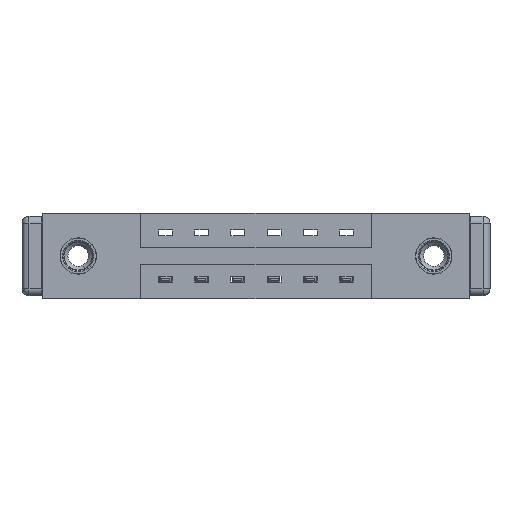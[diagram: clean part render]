
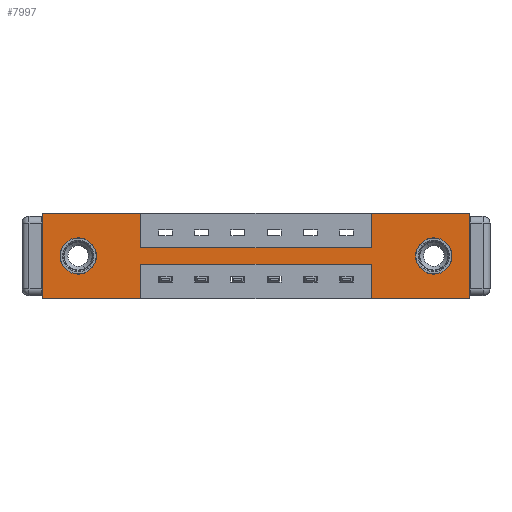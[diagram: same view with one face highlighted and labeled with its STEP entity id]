
A CAD part, front view. The second image highlights one B-rep face of the part: STEP entity #7997.
In plain terms, the highlighted planar face has unit normal (0, -1, 0).
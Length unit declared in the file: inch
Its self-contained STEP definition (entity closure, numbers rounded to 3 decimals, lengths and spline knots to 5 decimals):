
#38 = EDGE_CURVE ( 'NONE', #2394, #8816, #233, .T. ) ;
#136 = DIRECTION ( 'NONE',  ( 1., 0., 0. ) ) ;
#142 = DIRECTION ( 'NONE',  ( 0., 0., -1. ) ) ;
#158 = PLANE ( 'NONE',  #6622 ) ;
#172 = ORIENTED_EDGE ( 'NONE', *, *, #10269, .F. ) ;
#233 = LINE ( 'NONE', #5100, #368 ) ;
#368 = VECTOR ( 'NONE', #636, 39.37008 ) ;
#400 = VECTOR ( 'NONE', #8932, 39.37008 ) ;
#459 = CIRCLE ( 'NONE', #5070, 0.078 ) ;
#519 = ORIENTED_EDGE ( 'NONE', *, *, #772, .T. ) ;
#539 = ORIENTED_EDGE ( 'NONE', *, *, #7201, .F. ) ;
#636 = DIRECTION ( 'NONE',  ( 0., 0., 1. ) ) ;
#690 = VERTEX_POINT ( 'NONE', #1892 ) ;
#763 = DIRECTION ( 'NONE',  ( 0., 1., 0. ) ) ;
#772 = EDGE_CURVE ( 'NONE', #3120, #1529, #9039, .T. ) ;
#1170 = CARTESIAN_POINT ( 'NONE',  ( 0.425, 0., 0. ) ) ;
#1273 = ORIENTED_EDGE ( 'NONE', *, *, #7797, .F. ) ;
#1277 = ORIENTED_EDGE ( 'NONE', *, *, #1771, .F. ) ;
#1303 = ORIENTED_EDGE ( 'NONE', *, *, #38, .F. ) ;
#1448 = ORIENTED_EDGE ( 'NONE', *, *, #5580, .F. ) ;
#1529 = VERTEX_POINT ( 'NONE', #10705 ) ;
#1572 = DIRECTION ( 'NONE',  ( -1., 0., 0. ) ) ;
#1639 = CARTESIAN_POINT ( 'NONE',  ( 1.417, 0., -0.15 ) ) ;
#1703 = VERTEX_POINT ( 'NONE', #2415 ) ;
#1771 = EDGE_CURVE ( 'NONE', #8816, #7297, #5642, .T. ) ;
#1779 = CARTESIAN_POINT ( 'NONE',  ( 0., 0., 0. ) ) ;
#1783 = CARTESIAN_POINT ( 'NONE',  ( 0.425, 0., -0.15 ) ) ;
#1792 = FACE_BOUND ( 'NONE', #9631, .T. ) ;
#1835 = DIRECTION ( 'NONE',  ( 0., 0., -1. ) ) ;
#1892 = CARTESIAN_POINT ( 'NONE',  ( 0.155, 0., -0.107 ) ) ;
#1911 = EDGE_CURVE ( 'NONE', #3802, #2394, #8894, .T. ) ;
#1972 = CARTESIAN_POINT ( 'NONE',  ( 1.687, 0., -0.185 ) ) ;
#2100 = CARTESIAN_POINT ( 'NONE',  ( 0., 0., 0. ) ) ;
#2121 = VERTEX_POINT ( 'NONE', #7579 ) ;
#2150 = DIRECTION ( 'NONE',  ( 0., 0., 1. ) ) ;
#2299 = LINE ( 'NONE', #6321, #2576 ) ;
#2394 = VERTEX_POINT ( 'NONE', #1639 ) ;
#2415 = CARTESIAN_POINT ( 'NONE',  ( 1.417, 0., -0.37 ) ) ;
#2576 = VECTOR ( 'NONE', #3611, 39.37008 ) ;
#2641 = DIRECTION ( 'NONE',  ( 0., 0., -1. ) ) ;
#2748 = DIRECTION ( 'NONE',  ( 0., -1., 0. ) ) ;
#2850 = VERTEX_POINT ( 'NONE', #1170 ) ;
#2863 = DIRECTION ( 'NONE',  ( 0., 0., -1. ) ) ;
#3120 = VERTEX_POINT ( 'NONE', #9596 ) ;
#3240 = LINE ( 'NONE', #4805, #9347 ) ;
#3254 = LINE ( 'NONE', #8223, #7430 ) ;
#3289 = CARTESIAN_POINT ( 'NONE',  ( 0., 0., -0.37 ) ) ;
#3500 = CARTESIAN_POINT ( 'NONE',  ( 1.687, 0., -0.185 ) ) ;
#3555 = DIRECTION ( 'NONE',  ( 0., 0., 1. ) ) ;
#3592 = CARTESIAN_POINT ( 'NONE',  ( 0.425, 0., -0.37 ) ) ;
#3610 = VECTOR ( 'NONE', #8745, 39.37008 ) ;
#3611 = DIRECTION ( 'NONE',  ( -1., 0., 0. ) ) ;
#3703 = ORIENTED_EDGE ( 'NONE', *, *, #1911, .F. ) ;
#3747 = CARTESIAN_POINT ( 'NONE',  ( 0., 0., 0. ) ) ;
#3802 = VERTEX_POINT ( 'NONE', #10780 ) ;
#3962 = LINE ( 'NONE', #3289, #5983 ) ;
#4008 = CARTESIAN_POINT ( 'NONE',  ( 1.417, 0., -0.37 ) ) ;
#4165 = CARTESIAN_POINT ( 'NONE',  ( 1.417, 0., 0. ) ) ;
#4197 = LINE ( 'NONE', #4008, #3610 ) ;
#4304 = EDGE_CURVE ( 'NONE', #690, #10580, #10533, .T. ) ;
#4353 = ORIENTED_EDGE ( 'NONE', *, *, #11196, .T. ) ;
#4411 = DIRECTION ( 'NONE',  ( 0., 1., 0. ) ) ;
#4712 = CARTESIAN_POINT ( 'NONE',  ( 0.425, 0., -0.37 ) ) ;
#4805 = CARTESIAN_POINT ( 'NONE',  ( 1.842, 0., 0. ) ) ;
#5070 = AXIS2_PLACEMENT_3D ( 'NONE', #10750, #8829, #6153 ) ;
#5100 = CARTESIAN_POINT ( 'NONE',  ( 1.417, 0., 0. ) ) ;
#5190 = VECTOR ( 'NONE', #142, 39.37008 ) ;
#5369 = CARTESIAN_POINT ( 'NONE',  ( 0., 0., 0. ) ) ;
#5427 = VERTEX_POINT ( 'NONE', #8436 ) ;
#5496 = VECTOR ( 'NONE', #10717, 39.37008 ) ;
#5580 = EDGE_CURVE ( 'NONE', #2850, #3802, #3254, .T. ) ;
#5613 = LINE ( 'NONE', #2100, #9004 ) ;
#5642 = LINE ( 'NONE', #3747, #11686 ) ;
#5938 = LINE ( 'NONE', #11574, #5496 ) ;
#5973 = CARTESIAN_POINT ( 'NONE',  ( 0., 0., -0.37 ) ) ;
#5983 = VECTOR ( 'NONE', #1572, 39.37008 ) ;
#6144 = VERTEX_POINT ( 'NONE', #5369 ) ;
#6153 = DIRECTION ( 'NONE',  ( 0., 0., 1. ) ) ;
#6321 = CARTESIAN_POINT ( 'NONE',  ( 0., 0., -0.37 ) ) ;
#6336 = CARTESIAN_POINT ( 'NONE',  ( 0.155, 0., -0.263 ) ) ;
#6375 = FACE_OUTER_BOUND ( 'NONE', #10703, .T. ) ;
#6432 = AXIS2_PLACEMENT_3D ( 'NONE', #11595, #763, #3555 ) ;
#6466 = ORIENTED_EDGE ( 'NONE', *, *, #8921, .T. ) ;
#6527 = FACE_BOUND ( 'NONE', #11585, .T. ) ;
#6622 = AXIS2_PLACEMENT_3D ( 'NONE', #10886, #2748, #1835 ) ;
#6745 = EDGE_CURVE ( 'NONE', #7297, #5427, #3240, .T. ) ;
#6792 = DIRECTION ( 'NONE',  ( 1., 0., 0. ) ) ;
#7201 = EDGE_CURVE ( 'NONE', #2121, #8778, #8506, .T. ) ;
#7297 = VERTEX_POINT ( 'NONE', #11653 ) ;
#7430 = VECTOR ( 'NONE', #10011, 39.37008 ) ;
#7579 = CARTESIAN_POINT ( 'NONE',  ( 0.425, 0., -0.22 ) ) ;
#7640 = VECTOR ( 'NONE', #2150, 39.37008 ) ;
#7797 = EDGE_CURVE ( 'NONE', #9388, #2121, #5938, .T. ) ;
#7997 = ADVANCED_FACE ( 'NONE', ( #1792, #6527, #6375 ), #158, .T. ) ;
#8018 = ORIENTED_EDGE ( 'NONE', *, *, #8157, .F. ) ;
#8157 = EDGE_CURVE ( 'NONE', #1703, #9388, #4197, .T. ) ;
#8223 = CARTESIAN_POINT ( 'NONE',  ( 0.425, 0., 0. ) ) ;
#8436 = CARTESIAN_POINT ( 'NONE',  ( 1.842, 0., -0.37 ) ) ;
#8506 = LINE ( 'NONE', #4712, #5190 ) ;
#8715 = EDGE_CURVE ( 'NONE', #6144, #2850, #5613, .T. ) ;
#8745 = DIRECTION ( 'NONE',  ( 0., 0., 1. ) ) ;
#8778 = VERTEX_POINT ( 'NONE', #3592 ) ;
#8792 = EDGE_CURVE ( 'NONE', #8833, #6144, #11273, .T. ) ;
#8816 = VERTEX_POINT ( 'NONE', #4165 ) ;
#8829 = DIRECTION ( 'NONE',  ( 0., 1., 0. ) ) ;
#8833 = VERTEX_POINT ( 'NONE', #5973 ) ;
#8837 = ORIENTED_EDGE ( 'NONE', *, *, #6745, .F. ) ;
#8894 = LINE ( 'NONE', #1783, #400 ) ;
#8921 = EDGE_CURVE ( 'NONE', #1529, #3120, #9843, .T. ) ;
#8932 = DIRECTION ( 'NONE',  ( 1., 0., 0. ) ) ;
#9004 = VECTOR ( 'NONE', #6792, 39.37008 ) ;
#9027 = ORIENTED_EDGE ( 'NONE', *, *, #8792, .F. ) ;
#9039 = CIRCLE ( 'NONE', #9825, 0.078 ) ;
#9347 = VECTOR ( 'NONE', #2863, 39.37008 ) ;
#9388 = VERTEX_POINT ( 'NONE', #9684 ) ;
#9596 = CARTESIAN_POINT ( 'NONE',  ( 1.687, 0., -0.263 ) ) ;
#9631 = EDGE_LOOP ( 'NONE', ( #6466, #519 ) ) ;
#9678 = ORIENTED_EDGE ( 'NONE', *, *, #11363, .F. ) ;
#9684 = CARTESIAN_POINT ( 'NONE',  ( 1.417, 0., -0.22 ) ) ;
#9825 = AXIS2_PLACEMENT_3D ( 'NONE', #1972, #10078, #10939 ) ;
#9843 = CIRCLE ( 'NONE', #11695, 0.078 ) ;
#10011 = DIRECTION ( 'NONE',  ( 0., 0., -1. ) ) ;
#10078 = DIRECTION ( 'NONE',  ( 0., 1., 0. ) ) ;
#10093 = ORIENTED_EDGE ( 'NONE', *, *, #8715, .F. ) ;
#10269 = EDGE_CURVE ( 'NONE', #8778, #8833, #2299, .T. ) ;
#10533 = CIRCLE ( 'NONE', #6432, 0.078 ) ;
#10580 = VERTEX_POINT ( 'NONE', #6336 ) ;
#10703 = EDGE_LOOP ( 'NONE', ( #539, #1273, #8018, #9678, #8837, #1277, #1303, #3703, #1448, #10093, #9027, #172 ) ) ;
#10705 = CARTESIAN_POINT ( 'NONE',  ( 1.687, 0., -0.107 ) ) ;
#10717 = DIRECTION ( 'NONE',  ( -1., 0., 0. ) ) ;
#10750 = CARTESIAN_POINT ( 'NONE',  ( 0.155, 0., -0.185 ) ) ;
#10780 = CARTESIAN_POINT ( 'NONE',  ( 0.425, 0., -0.15 ) ) ;
#10886 = CARTESIAN_POINT ( 'NONE',  ( 0., 0., -0.37 ) ) ;
#10934 = ORIENTED_EDGE ( 'NONE', *, *, #4304, .T. ) ;
#10939 = DIRECTION ( 'NONE',  ( 0., 0., -1. ) ) ;
#11196 = EDGE_CURVE ( 'NONE', #10580, #690, #459, .T. ) ;
#11273 = LINE ( 'NONE', #1779, #7640 ) ;
#11363 = EDGE_CURVE ( 'NONE', #5427, #1703, #3962, .T. ) ;
#11574 = CARTESIAN_POINT ( 'NONE',  ( 0.425, 0., -0.22 ) ) ;
#11585 = EDGE_LOOP ( 'NONE', ( #10934, #4353 ) ) ;
#11595 = CARTESIAN_POINT ( 'NONE',  ( 0.155, 0., -0.185 ) ) ;
#11653 = CARTESIAN_POINT ( 'NONE',  ( 1.842, 0., 0. ) ) ;
#11686 = VECTOR ( 'NONE', #136, 39.37008 ) ;
#11695 = AXIS2_PLACEMENT_3D ( 'NONE', #3500, #4411, #2641 ) ;
